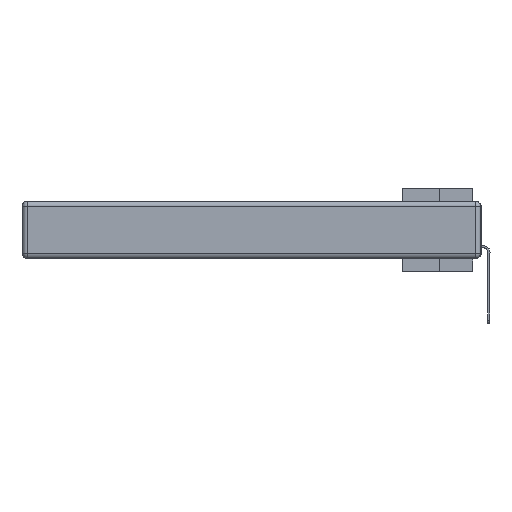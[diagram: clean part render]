
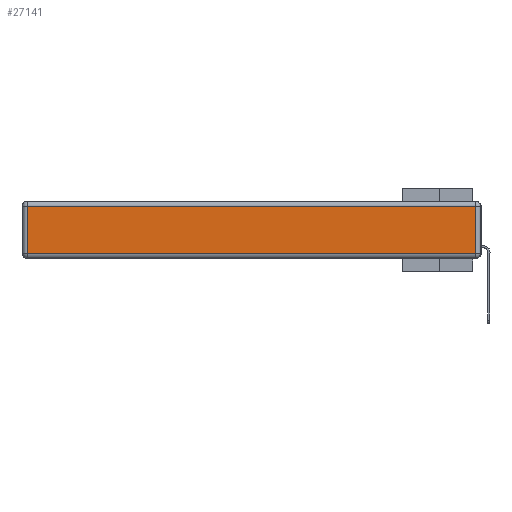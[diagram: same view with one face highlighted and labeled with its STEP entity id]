
A CAD part, left-side view. The second image highlights one B-rep face of the part: STEP entity #27141.
In plain terms, the highlighted planar face has unit normal (-1, 0, 0).
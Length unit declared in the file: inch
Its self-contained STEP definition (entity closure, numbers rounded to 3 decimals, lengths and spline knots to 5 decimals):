
#1633 = ORIENTED_EDGE ( 'NONE', *, *, #22410, .T. ) ;
#1975 = CARTESIAN_POINT ( 'NONE',  ( 0., 0.03, -0.313 ) ) ;
#2074 = CARTESIAN_POINT ( 'NONE',  ( 0., 0.03, -0.343 ) ) ;
#2642 = VECTOR ( 'NONE', #12416, 39.37008 ) ;
#3027 = VECTOR ( 'NONE', #26128, 39.37008 ) ;
#3261 = CARTESIAN_POINT ( 'NONE',  ( 0., 0., -0.313 ) ) ;
#4985 = EDGE_CURVE ( 'NONE', #19886, #9308, #19433, .T. ) ;
#6137 = VECTOR ( 'NONE', #18749, 39.37008 ) ;
#8577 = EDGE_LOOP ( 'NONE', ( #25764, #1633, #24064, #11866 ) ) ;
#9308 = VERTEX_POINT ( 'NONE', #26947 ) ;
#11502 = PLANE ( 'NONE',  #16278 ) ;
#11866 = ORIENTED_EDGE ( 'NONE', *, *, #4985, .T. ) ;
#12416 = DIRECTION ( 'NONE',  ( 0., 1., 0. ) ) ;
#16278 = AXIS2_PLACEMENT_3D ( 'NONE', #16588, #28118, #18652 ) ;
#16588 = CARTESIAN_POINT ( 'NONE',  ( 0., 0., -0.343 ) ) ;
#17398 = CARTESIAN_POINT ( 'NONE',  ( 0., 2.75, -0.03 ) ) ;
#17902 = EDGE_CURVE ( 'NONE', #9308, #22425, #21347, .T. ) ;
#18652 = DIRECTION ( 'NONE',  ( 0., 0., 1. ) ) ;
#18749 = DIRECTION ( 'NONE',  ( 0., 0., 1. ) ) ;
#18788 = EDGE_CURVE ( 'NONE', #21821, #19886, #19050, .T. ) ;
#19050 = LINE ( 'NONE', #17398, #2642 ) ;
#19433 = LINE ( 'NONE', #26226, #3027 ) ;
#19886 = VERTEX_POINT ( 'NONE', #28925 ) ;
#19926 = DIRECTION ( 'NONE',  ( 0., -1., 0. ) ) ;
#21347 = LINE ( 'NONE', #3261, #27665 ) ;
#21821 = VERTEX_POINT ( 'NONE', #22946 ) ;
#22410 = EDGE_CURVE ( 'NONE', #22425, #21821, #26227, .T. ) ;
#22425 = VERTEX_POINT ( 'NONE', #1975 ) ;
#22946 = CARTESIAN_POINT ( 'NONE',  ( 0., 0.03, -0.03 ) ) ;
#24064 = ORIENTED_EDGE ( 'NONE', *, *, #18788, .T. ) ;
#25708 = FACE_OUTER_BOUND ( 'NONE', #8577, .T. ) ;
#25764 = ORIENTED_EDGE ( 'NONE', *, *, #17902, .T. ) ;
#26128 = DIRECTION ( 'NONE',  ( 0., 0., -1. ) ) ;
#26226 = CARTESIAN_POINT ( 'NONE',  ( 0., 2.72, -0.343 ) ) ;
#26227 = LINE ( 'NONE', #2074, #6137 ) ;
#26947 = CARTESIAN_POINT ( 'NONE',  ( 0., 2.72, -0.313 ) ) ;
#27141 = ADVANCED_FACE ( 'NONE', ( #25708 ), #11502, .T. ) ;
#27665 = VECTOR ( 'NONE', #19926, 39.37008 ) ;
#28118 = DIRECTION ( 'NONE',  ( -1., 0., 0. ) ) ;
#28925 = CARTESIAN_POINT ( 'NONE',  ( 0., 2.72, -0.03 ) ) ;
